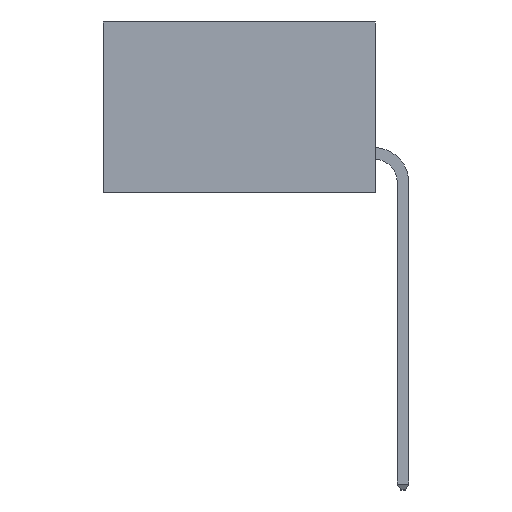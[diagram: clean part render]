
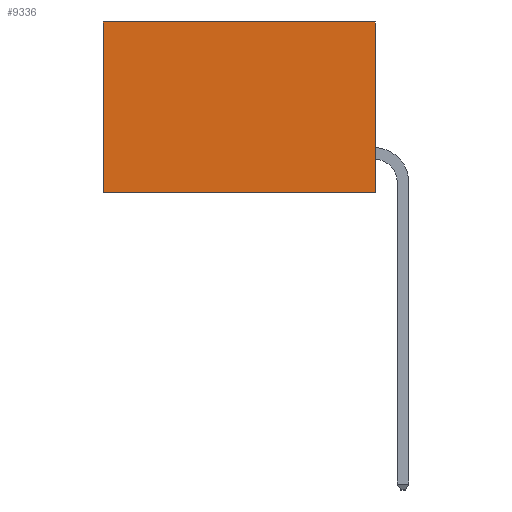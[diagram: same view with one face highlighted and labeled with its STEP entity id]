
A CAD part, left-side view. The second image highlights one B-rep face of the part: STEP entity #9336.
In plain terms, the highlighted planar face has unit normal (-1, 0, 0).
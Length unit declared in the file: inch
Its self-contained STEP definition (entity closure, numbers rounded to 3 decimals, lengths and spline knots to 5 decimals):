
#1188 = VECTOR ( 'NONE', #8443, 39.37008 ) ;
#1981 = ORIENTED_EDGE ( 'NONE', *, *, #14582, .T. ) ;
#2073 = CARTESIAN_POINT ( 'NONE',  ( 0.277, 0.59, -0.37 ) ) ;
#2994 = EDGE_CURVE ( 'NONE', #13252, #10757, #4609, .T. ) ;
#3801 = CARTESIAN_POINT ( 'NONE',  ( 0.277, 0., 0. ) ) ;
#4609 = LINE ( 'NONE', #15065, #8316 ) ;
#5037 = DIRECTION ( 'NONE',  ( 0., 0., -1. ) ) ;
#5492 = CARTESIAN_POINT ( 'NONE',  ( 0.277, 0., -0.37 ) ) ;
#5826 = EDGE_CURVE ( 'NONE', #10757, #10010, #9969, .T. ) ;
#6865 = LINE ( 'NONE', #3801, #10551 ) ;
#6972 = VERTEX_POINT ( 'NONE', #7405 ) ;
#7405 = CARTESIAN_POINT ( 'NONE',  ( 0.277, 0.59, 0. ) ) ;
#8316 = VECTOR ( 'NONE', #15040, 39.37008 ) ;
#8443 = DIRECTION ( 'NONE',  ( 0., 0., -1. ) ) ;
#9336 = ADVANCED_FACE ( 'NONE', ( #10707 ), #10559, .F. ) ;
#9343 = ORIENTED_EDGE ( 'NONE', *, *, #12086, .T. ) ;
#9393 = ORIENTED_EDGE ( 'NONE', *, *, #2994, .F. ) ;
#9544 = VECTOR ( 'NONE', #10448, 39.37008 ) ;
#9969 = LINE ( 'NONE', #10328, #9544 ) ;
#10010 = VERTEX_POINT ( 'NONE', #2073 ) ;
#10328 = CARTESIAN_POINT ( 'NONE',  ( 0.277, 0., -0.37 ) ) ;
#10448 = DIRECTION ( 'NONE',  ( 0., 1., 0. ) ) ;
#10551 = VECTOR ( 'NONE', #12098, 39.37008 ) ;
#10559 = PLANE ( 'NONE',  #17403 ) ;
#10707 = FACE_OUTER_BOUND ( 'NONE', #15929, .T. ) ;
#10757 = VERTEX_POINT ( 'NONE', #5492 ) ;
#11930 = CARTESIAN_POINT ( 'NONE',  ( 0.277, 0., -0.37 ) ) ;
#12086 = EDGE_CURVE ( 'NONE', #13252, #6972, #6865, .T. ) ;
#12098 = DIRECTION ( 'NONE',  ( 0., 1., 0. ) ) ;
#12367 = LINE ( 'NONE', #16619, #1188 ) ;
#13252 = VERTEX_POINT ( 'NONE', #14398 ) ;
#13322 = DIRECTION ( 'NONE',  ( 1., 0., 0. ) ) ;
#14398 = CARTESIAN_POINT ( 'NONE',  ( 0.277, 0., 0. ) ) ;
#14582 = EDGE_CURVE ( 'NONE', #6972, #10010, #12367, .T. ) ;
#15040 = DIRECTION ( 'NONE',  ( 0., 0., -1. ) ) ;
#15065 = CARTESIAN_POINT ( 'NONE',  ( 0.277, 0., -0.37 ) ) ;
#15929 = EDGE_LOOP ( 'NONE', ( #1981, #17452, #9393, #9343 ) ) ;
#16619 = CARTESIAN_POINT ( 'NONE',  ( 0.277, 0.59, -0.37 ) ) ;
#17403 = AXIS2_PLACEMENT_3D ( 'NONE', #11930, #13322, #5037 ) ;
#17452 = ORIENTED_EDGE ( 'NONE', *, *, #5826, .F. ) ;
